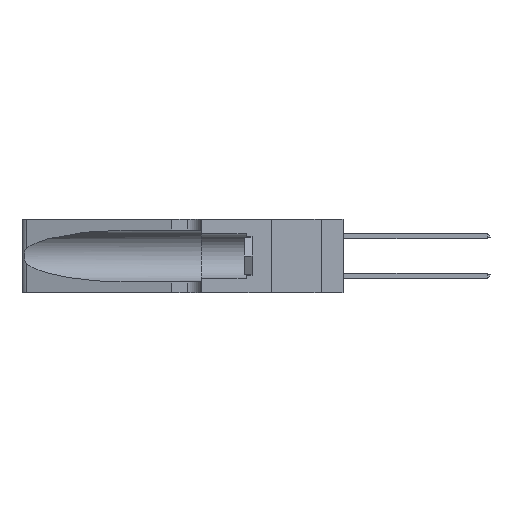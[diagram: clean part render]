
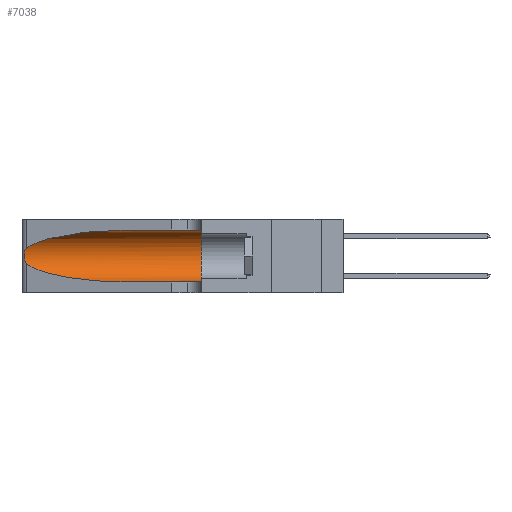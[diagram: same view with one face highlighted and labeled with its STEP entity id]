
A CAD part, left-side view. The second image highlights one B-rep face of the part: STEP entity #7038.
In plain terms, the highlighted cylindrical face has radius 3.308 mm (diameter 6.617 mm), a partial arc.
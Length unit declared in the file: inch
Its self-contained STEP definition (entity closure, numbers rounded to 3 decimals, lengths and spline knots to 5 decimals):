
#344 = CARTESIAN_POINT ( 'NONE',  ( 0.25487, 1.22718, 0.22369 ) ) ;
#1426 = VERTEX_POINT ( 'NONE', #344 ) ;
#1816 = CARTESIAN_POINT ( 'NONE',  ( 0.25555, 1.22994, 0.2215 ) ) ;
#1897 = CARTESIAN_POINT ( 'NONE',  ( 0.26075, 1.23896, 0.178 ) ) ;
#3209 = ORIENTED_EDGE ( 'NONE', *, *, #5480, .T. ) ;
#3447 = ORIENTED_EDGE ( 'NONE', *, *, #24337, .T. ) ;
#3712 = CYLINDRICAL_SURFACE ( 'NONE', #8198, 0.13025 ) ;
#3790 = ORIENTED_EDGE ( 'NONE', *, *, #10752, .T. ) ;
#3975 = CARTESIAN_POINT ( 'NONE',  ( 0.25856, 1.23593, 0.16098 ) ) ;
#4013 = CARTESIAN_POINT ( 'NONE',  ( 0.1305, 1.61858, 0.185 ) ) ;
#4622 = CIRCLE ( 'NONE', #5845, 0.13025 ) ;
#5238 = VECTOR ( 'NONE', #24018, 39.37008 ) ;
#5480 = EDGE_CURVE ( 'NONE', #1426, #6138, #11112, .T. ) ;
#5845 = AXIS2_PLACEMENT_3D ( 'NONE', #18062, #6157, #20063 ) ;
#5855 = ORIENTED_EDGE ( 'NONE', *, *, #7702, .F. ) ;
#6019 = DIRECTION ( 'NONE',  ( 0., 0., -1. ) ) ;
#6066 = CARTESIAN_POINT ( 'NONE',  ( 0.25639, 1.23186, 0.15144 ) ) ;
#6138 = VERTEX_POINT ( 'NONE', #9829 ) ;
#6157 = DIRECTION ( 'NONE',  ( 0., 1., 0. ) ) ;
#6273 = CARTESIAN_POINT ( 'NONE',  ( 0.1305, 0.35, 0.05475 ) ) ;
#7038 = ADVANCED_FACE ( 'NONE', ( #15007 ), #3712, .F. ) ;
#7265 = CARTESIAN_POINT ( 'NONE',  ( 0.1305, 0.72297, 0.05475 ) ) ;
#7702 = EDGE_CURVE ( 'NONE', #8089, #18322, #4622, .T. ) ;
#8089 = VERTEX_POINT ( 'NONE', #19094 ) ;
#8097 = CARTESIAN_POINT ( 'NONE',  ( 0.25487, 1.22718, 0.14631 ) ) ;
#8198 = AXIS2_PLACEMENT_3D ( 'NONE', #4013, #20010, #6019 ) ;
#8909 = CARTESIAN_POINT ( 'NONE',  ( 0.2373, 1.15595, 0.28018 ) ) ;
#9305 = ORIENTED_EDGE ( 'NONE', *, *, #21028, .F. ) ;
#9575 = ORIENTED_EDGE ( 'NONE', *, *, #16639, .T. ) ;
#9701 = VERTEX_POINT ( 'NONE', #16411 ) ;
#9829 = CARTESIAN_POINT ( 'NONE',  ( 0.25487, 1.22718, 0.14631 ) ) ;
#10034 = CARTESIAN_POINT ( 'NONE',  ( 0.25639, 1.23184, 0.21858 ) ) ;
#10188 = CARTESIAN_POINT ( 'NONE',  ( 0.1305, 1.61858, 0.05475 ) ) ;
#10752 = EDGE_CURVE ( 'NONE', #6138, #17071, #23021, .T. ) ;
#11112 = B_SPLINE_CURVE_WITH_KNOTS ( 'NONE', 3,
 ( #25757, #1816, #10034, #23869, #12024, #25841, #13975, #1897, #15976, #3975, #17969, #6066, #19967, #8097 ),
 .UNSPECIFIED., .F., .F.,
 ( 4, 2, 2, 2, 2, 2, 4 ),
 ( 0., 0.00027, 0.00053, 0.00107, 0.0016, 0.00187, 0.00214 ),
 .UNSPECIFIED. ) ;
#11403 = DIRECTION ( 'NONE',  ( 0., -1., 0. ) ) ;
#12024 = CARTESIAN_POINT ( 'NONE',  ( 0.25854, 1.2359, 0.20912 ) ) ;
#12789 = CARTESIAN_POINT ( 'NONE',  ( 0.1305, 0.72297, 0.31525 ) ) ;
#13975 = CARTESIAN_POINT ( 'NONE',  ( 0.26075, 1.23896, 0.19203 ) ) ;
#15007 = FACE_OUTER_BOUND ( 'NONE', #17397, .T. ) ;
#15976 = CARTESIAN_POINT ( 'NONE',  ( 0.26017, 1.23833, 0.17102 ) ) ;
#16411 = CARTESIAN_POINT ( 'NONE',  ( 0.1305, 0.72297, 0.31525 ) ) ;
#16472 =( BOUNDED_CURVE ( )  B_SPLINE_CURVE ( 3, ( #12789, #16758, #8909, #22780 ),
 .UNSPECIFIED., .F., .T. ) 
 B_SPLINE_CURVE_WITH_KNOTS ( ( 4, 4 ),
 ( 1.5708, 2.84003 ),
 .UNSPECIFIED. ) 
 CURVE ( )  GEOMETRIC_REPRESENTATION_ITEM ( )  RATIONAL_B_SPLINE_CURVE ( ( 1., 0.87, 0.87, 1. ) ) 
 REPRESENTATION_ITEM ( '' )  );
#16639 = EDGE_CURVE ( 'NONE', #9701, #1426, #16472, .T. ) ;
#16758 = CARTESIAN_POINT ( 'NONE',  ( 0.18966, 0.96281, 0.31525 ) ) ;
#17071 = VERTEX_POINT ( 'NONE', #20060 ) ;
#17148 = CARTESIAN_POINT ( 'NONE',  ( 0.2373, 1.15595, 0.08982 ) ) ;
#17397 = EDGE_LOOP ( 'NONE', ( #9575, #3209, #3790, #3447, #5855, #9305 ) ) ;
#17969 = CARTESIAN_POINT ( 'NONE',  ( 0.25789, 1.23486, 0.15765 ) ) ;
#18062 = CARTESIAN_POINT ( 'NONE',  ( 0.1305, 0.35, 0.185 ) ) ;
#18322 = VERTEX_POINT ( 'NONE', #6273 ) ;
#19094 = CARTESIAN_POINT ( 'NONE',  ( 0.1305, 0.35, 0.31525 ) ) ;
#19146 = CARTESIAN_POINT ( 'NONE',  ( 0.18966, 0.96281, 0.05475 ) ) ;
#19967 = CARTESIAN_POINT ( 'NONE',  ( 0.25555, 1.22993, 0.14849 ) ) ;
#20010 = DIRECTION ( 'NONE',  ( 0., -1., 0. ) ) ;
#20024 = VECTOR ( 'NONE', #11403, 39.37008 ) ;
#20060 = CARTESIAN_POINT ( 'NONE',  ( 0.1305, 0.72297, 0.05475 ) ) ;
#20063 = DIRECTION ( 'NONE',  ( 0., 0., 1. ) ) ;
#21028 = EDGE_CURVE ( 'NONE', #9701, #8089, #25296, .T. ) ;
#21348 = CARTESIAN_POINT ( 'NONE',  ( 0.1305, 1.61858, 0.31525 ) ) ;
#22780 = CARTESIAN_POINT ( 'NONE',  ( 0.25487, 1.22718, 0.22369 ) ) ;
#23021 =( BOUNDED_CURVE ( )  B_SPLINE_CURVE ( 3, ( #23075, #17148, #19146, #7265 ),
 .UNSPECIFIED., .F., .F. ) 
 B_SPLINE_CURVE_WITH_KNOTS ( ( 4, 4 ),
 ( 3.44316, 4.71239 ),
 .UNSPECIFIED. ) 
 CURVE ( )  GEOMETRIC_REPRESENTATION_ITEM ( )  RATIONAL_B_SPLINE_CURVE ( ( 1., 0.87, 0.87, 1. ) ) 
 REPRESENTATION_ITEM ( '' )  );
#23075 = CARTESIAN_POINT ( 'NONE',  ( 0.25487, 1.22718, 0.14631 ) ) ;
#23869 = CARTESIAN_POINT ( 'NONE',  ( 0.25787, 1.23484, 0.2124 ) ) ;
#24018 = DIRECTION ( 'NONE',  ( 0., -1., 0. ) ) ;
#24337 = EDGE_CURVE ( 'NONE', #17071, #18322, #25155, .T. ) ;
#25155 = LINE ( 'NONE', #10188, #5238 ) ;
#25296 = LINE ( 'NONE', #21348, #20024 ) ;
#25757 = CARTESIAN_POINT ( 'NONE',  ( 0.25487, 1.22718, 0.22369 ) ) ;
#25841 = CARTESIAN_POINT ( 'NONE',  ( 0.26018, 1.23835, 0.19895 ) ) ;
